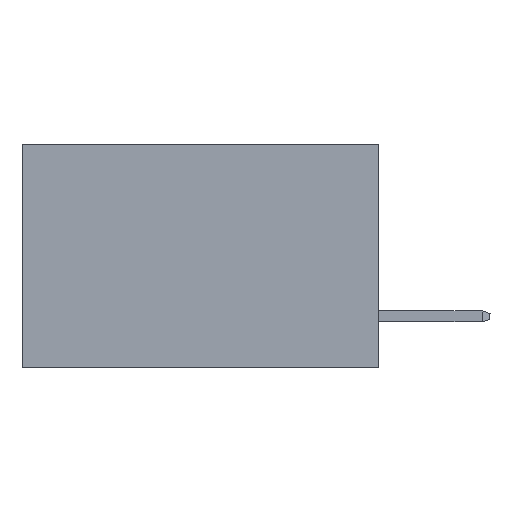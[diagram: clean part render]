
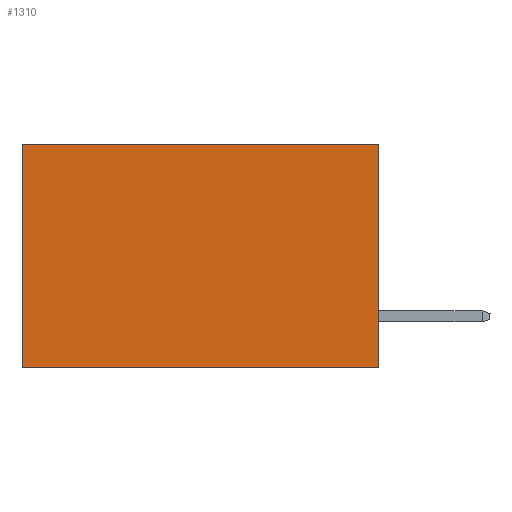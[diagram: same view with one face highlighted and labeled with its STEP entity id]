
A CAD part, left-side view. The second image highlights one B-rep face of the part: STEP entity #1310.
In plain terms, the highlighted planar face has unit normal (-1, 0, 0).
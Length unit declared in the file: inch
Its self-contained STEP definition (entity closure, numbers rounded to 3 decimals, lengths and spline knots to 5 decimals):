
#27 = DIRECTION ( 'NONE',  ( 0., 1., 0. ) ) ;
#345 = DIRECTION ( 'NONE',  ( 0., 1., 0. ) ) ;
#554 = DIRECTION ( 'NONE',  ( 0., 0., -1. ) ) ;
#1038 = CARTESIAN_POINT ( 'NONE',  ( 0.277, 0., -0.37 ) ) ;
#1295 = VECTOR ( 'NONE', #4009, 39.37008 ) ;
#1310 = ADVANCED_FACE ( 'NONE', ( #13238 ), #9692, .F. ) ;
#1402 = VERTEX_POINT ( 'NONE', #6034 ) ;
#1437 = DIRECTION ( 'NONE',  ( 0., 0., -1. ) ) ;
#1839 = EDGE_CURVE ( 'NONE', #10740, #1402, #6954, .T. ) ;
#1849 = VERTEX_POINT ( 'NONE', #7292 ) ;
#2019 = VECTOR ( 'NONE', #1437, 39.37008 ) ;
#3555 = DIRECTION ( 'NONE',  ( 1., 0., 0. ) ) ;
#4009 = DIRECTION ( 'NONE',  ( 0., 0., -1. ) ) ;
#4300 = AXIS2_PLACEMENT_3D ( 'NONE', #6592, #3555, #554 ) ;
#4568 = VECTOR ( 'NONE', #345, 39.37008 ) ;
#4954 = CARTESIAN_POINT ( 'NONE',  ( 0.277, 0.59, 0. ) ) ;
#5729 = CARTESIAN_POINT ( 'NONE',  ( 0.277, 0.59, -0.37 ) ) ;
#6028 = CARTESIAN_POINT ( 'NONE',  ( 0.277, 0., -0.37 ) ) ;
#6034 = CARTESIAN_POINT ( 'NONE',  ( 0.277, 0.59, -0.37 ) ) ;
#6373 = ORIENTED_EDGE ( 'NONE', *, *, #11957, .F. ) ;
#6592 = CARTESIAN_POINT ( 'NONE',  ( 0.277, 0., -0.37 ) ) ;
#6776 = CARTESIAN_POINT ( 'NONE',  ( 0.277, 0., 0. ) ) ;
#6954 = LINE ( 'NONE', #5729, #1295 ) ;
#7181 = LINE ( 'NONE', #6028, #4568 ) ;
#7292 = CARTESIAN_POINT ( 'NONE',  ( 0.277, 0., 0. ) ) ;
#7407 = ORIENTED_EDGE ( 'NONE', *, *, #7686, .F. ) ;
#7686 = EDGE_CURVE ( 'NONE', #1849, #11167, #13582, .T. ) ;
#7876 = CARTESIAN_POINT ( 'NONE',  ( 0.277, 0., -0.37 ) ) ;
#8084 = ORIENTED_EDGE ( 'NONE', *, *, #13245, .T. ) ;
#8264 = VECTOR ( 'NONE', #27, 39.37008 ) ;
#9692 = PLANE ( 'NONE',  #4300 ) ;
#10740 = VERTEX_POINT ( 'NONE', #4954 ) ;
#11167 = VERTEX_POINT ( 'NONE', #7876 ) ;
#11727 = ORIENTED_EDGE ( 'NONE', *, *, #1839, .T. ) ;
#11742 = LINE ( 'NONE', #6776, #8264 ) ;
#11848 = EDGE_LOOP ( 'NONE', ( #11727, #6373, #7407, #8084 ) ) ;
#11957 = EDGE_CURVE ( 'NONE', #11167, #1402, #7181, .T. ) ;
#13238 = FACE_OUTER_BOUND ( 'NONE', #11848, .T. ) ;
#13245 = EDGE_CURVE ( 'NONE', #1849, #10740, #11742, .T. ) ;
#13582 = LINE ( 'NONE', #1038, #2019 ) ;
